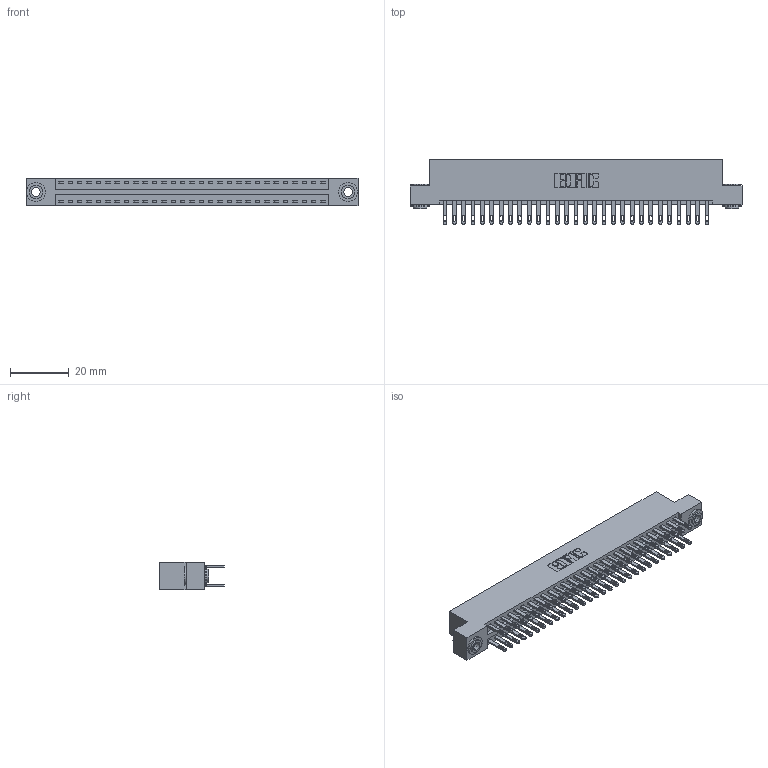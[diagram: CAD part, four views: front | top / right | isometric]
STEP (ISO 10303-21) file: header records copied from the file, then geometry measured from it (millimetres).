
FILE_DESCRIPTION (( 'STEP AP203' ), '1' );
FILE_NAME ('346-058-500-203.STEP', '2022-05-21T07:18:47', ( '' ), ( '' ), 'SwSTEP 2.0', 'SolidWorks 2020', '' );
FILE_SCHEMA (( 'CONFIG_CONTROL_DESIGN' ));
Length unit declared in the file: inch
Products named in the file (4): 345-292-001_345-293-100; 345-250-002_345-250-002-102; 346 Part_Flush Mounting Lugs - 0.156 Dia-TH; 346-058-500-203
Assembly tree (61 placements, depth 2):
  346-058-500-203
    346 Part_Flush Mounting Lugs - 0.156 Dia-TH
    345-292-001_345-293-100  x58
    345-250-002_345-250-002-102  x2
Bounding box: 112.65 x 21.84 x 9.4 mm (x, y, z)
Volume: 11062.2 mm3; surface area: 15857.3 mm2
Topology: 61 solids, 61 shells, 2958 faces, 8967 edges, 5974 vertices
Faces by surface type: plane 1782, cylinder 1168, cone 8
Entity records: 21672 total; most frequent: CARTESIAN_POINT 3569, ORIENTED_EDGE 3494, DIRECTION 3229, EDGE_CURVE 1747, LINE 1471, VECTOR 1471, VERTEX_POINT 1162, AXIS2_PLACEMENT_3D 879
